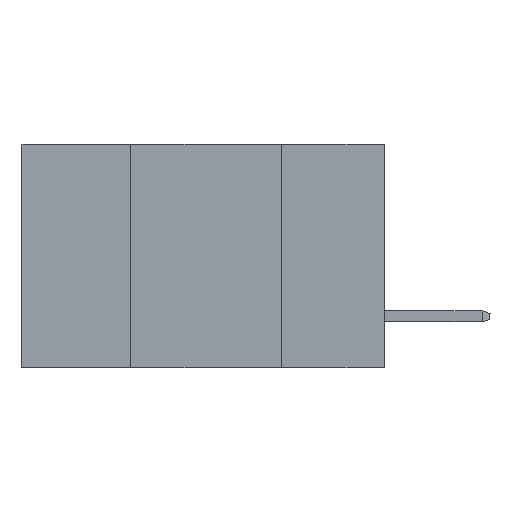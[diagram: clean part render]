
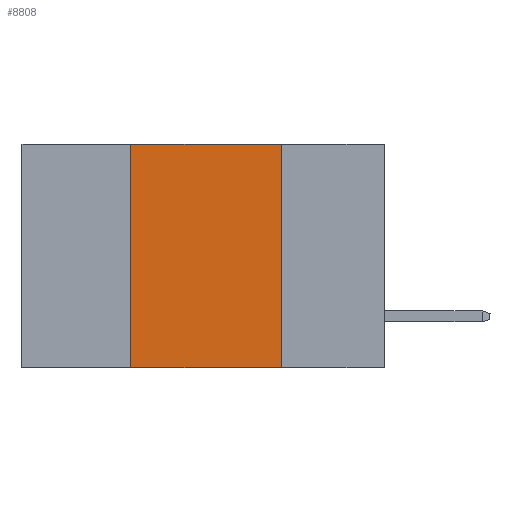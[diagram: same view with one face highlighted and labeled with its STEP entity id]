
A CAD part, left-side view. The second image highlights one B-rep face of the part: STEP entity #8808.
In plain terms, the highlighted planar face has unit normal (-1, 0, 0).
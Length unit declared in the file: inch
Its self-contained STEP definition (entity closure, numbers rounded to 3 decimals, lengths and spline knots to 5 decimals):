
#125 = LINE ( 'NONE', #3437, #3355 ) ;
#311 = EDGE_LOOP ( 'NONE', ( #1870, #1285, #9027, #4987 ) ) ;
#857 = DIRECTION ( 'NONE',  ( 0., 0., -1. ) ) ;
#895 = CARTESIAN_POINT ( 'NONE',  ( 0., 0.42, -0.37 ) ) ;
#1042 = VECTOR ( 'NONE', #10194, 39.37008 ) ;
#1085 = CARTESIAN_POINT ( 'NONE',  ( 0., 0.17, 0. ) ) ;
#1106 = VERTEX_POINT ( 'NONE', #7270 ) ;
#1285 = ORIENTED_EDGE ( 'NONE', *, *, #1693, .F. ) ;
#1300 = DIRECTION ( 'NONE',  ( 0., -1., 0. ) ) ;
#1364 = EDGE_CURVE ( 'NONE', #1106, #5055, #8683, .T. ) ;
#1663 = EDGE_CURVE ( 'NONE', #1106, #1938, #1875, .T. ) ;
#1693 = EDGE_CURVE ( 'NONE', #1938, #7170, #125, .T. ) ;
#1870 = ORIENTED_EDGE ( 'NONE', *, *, #8906, .F. ) ;
#1875 = LINE ( 'NONE', #895, #10435 ) ;
#1938 = VERTEX_POINT ( 'NONE', #10619 ) ;
#2106 = CARTESIAN_POINT ( 'NONE',  ( 0., 0.6, -0.37 ) ) ;
#2481 = FACE_OUTER_BOUND ( 'NONE', #311, .T. ) ;
#3355 = VECTOR ( 'NONE', #9193, 39.37008 ) ;
#3437 = CARTESIAN_POINT ( 'NONE',  ( 0., 0.6, 0. ) ) ;
#4190 = DIRECTION ( 'NONE',  ( 1., 0., 0. ) ) ;
#4412 = LINE ( 'NONE', #8564, #1042 ) ;
#4987 = ORIENTED_EDGE ( 'NONE', *, *, #1364, .T. ) ;
#5055 = VERTEX_POINT ( 'NONE', #10026 ) ;
#5863 = CARTESIAN_POINT ( 'NONE',  ( 0., 0.6, 0. ) ) ;
#6765 = DIRECTION ( 'NONE',  ( 0., 0., 1. ) ) ;
#7170 = VERTEX_POINT ( 'NONE', #1085 ) ;
#7270 = CARTESIAN_POINT ( 'NONE',  ( 0., 0.42, -0.37 ) ) ;
#8245 = PLANE ( 'NONE',  #9838 ) ;
#8564 = CARTESIAN_POINT ( 'NONE',  ( 0., 0.17, -0.37 ) ) ;
#8683 = LINE ( 'NONE', #2106, #10057 ) ;
#8808 = ADVANCED_FACE ( 'NONE', ( #2481 ), #8245, .F. ) ;
#8906 = EDGE_CURVE ( 'NONE', #7170, #5055, #4412, .T. ) ;
#9027 = ORIENTED_EDGE ( 'NONE', *, *, #1663, .F. ) ;
#9193 = DIRECTION ( 'NONE',  ( 0., -1., 0. ) ) ;
#9838 = AXIS2_PLACEMENT_3D ( 'NONE', #5863, #4190, #857 ) ;
#10026 = CARTESIAN_POINT ( 'NONE',  ( 0., 0.17, -0.37 ) ) ;
#10057 = VECTOR ( 'NONE', #1300, 39.37008 ) ;
#10194 = DIRECTION ( 'NONE',  ( 0., 0., -1. ) ) ;
#10435 = VECTOR ( 'NONE', #6765, 39.37008 ) ;
#10619 = CARTESIAN_POINT ( 'NONE',  ( 0., 0.42, 0. ) ) ;
